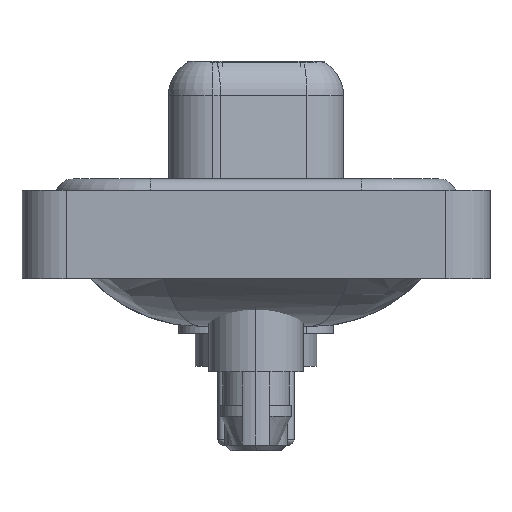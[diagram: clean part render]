
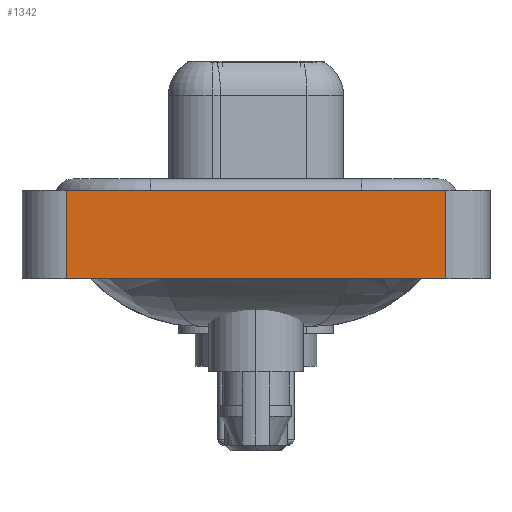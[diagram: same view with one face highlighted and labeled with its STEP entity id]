
A CAD part, left-side view. The second image highlights one B-rep face of the part: STEP entity #1342.
In plain terms, the highlighted planar face has unit normal (-1, 0, 0).
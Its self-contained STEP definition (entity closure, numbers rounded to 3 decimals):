
#61 = VERTEX_POINT ( 'NONE', #8482 ) ;
#891 = EDGE_LOOP ( 'NONE', ( #1955, #5107, #23149, #19632 ) ) ;
#1128 = EDGE_CURVE ( 'NONE', #61, #12502, #7749, .T. ) ;
#1342 = ADVANCED_FACE ( 'NONE', ( #24289 ), #12551, .T. ) ;
#1526 = VECTOR ( 'NONE', #23665, 1000. ) ;
#1574 = CARTESIAN_POINT ( 'NONE',  ( -7.35, -8.55, 0.4 ) ) ;
#1955 = ORIENTED_EDGE ( 'NONE', *, *, #8724, .T. ) ;
#3201 = CARTESIAN_POINT ( 'NONE',  ( -7.35, -8.55, -3.6 ) ) ;
#4560 = CARTESIAN_POINT ( 'NONE',  ( -7.35, 8.55, 0.4 ) ) ;
#4996 = LINE ( 'NONE', #3201, #21422 ) ;
#5107 = ORIENTED_EDGE ( 'NONE', *, *, #14108, .F. ) ;
#5480 = DIRECTION ( 'NONE',  ( 0., 0., 1. ) ) ;
#7309 = CARTESIAN_POINT ( 'NONE',  ( -7.35, -8.55, -3.6 ) ) ;
#7749 = LINE ( 'NONE', #10145, #1526 ) ;
#8010 = CARTESIAN_POINT ( 'NONE',  ( -7.35, -8.55, 0.4 ) ) ;
#8261 = LINE ( 'NONE', #8010, #17366 ) ;
#8482 = CARTESIAN_POINT ( 'NONE',  ( -7.35, 8.55, -3.6 ) ) ;
#8724 = EDGE_CURVE ( 'NONE', #21779, #14314, #4996, .T. ) ;
#10037 = DIRECTION ( 'NONE',  ( 0., -1., 0. ) ) ;
#10145 = CARTESIAN_POINT ( 'NONE',  ( -7.35, 8.55, -3.6 ) ) ;
#12502 = VERTEX_POINT ( 'NONE', #4560 ) ;
#12551 = PLANE ( 'NONE',  #16206 ) ;
#13520 = LINE ( 'NONE', #19129, #15244 ) ;
#14108 = EDGE_CURVE ( 'NONE', #12502, #14314, #8261, .T. ) ;
#14314 = VERTEX_POINT ( 'NONE', #1574 ) ;
#15244 = VECTOR ( 'NONE', #23342, 1000. ) ;
#16087 = EDGE_CURVE ( 'NONE', #61, #21779, #13520, .T. ) ;
#16206 = AXIS2_PLACEMENT_3D ( 'NONE', #22251, #16640, #24420 ) ;
#16640 = DIRECTION ( 'NONE',  ( -1., 0., 0. ) ) ;
#17366 = VECTOR ( 'NONE', #10037, 1000. ) ;
#19129 = CARTESIAN_POINT ( 'NONE',  ( -7.35, -8.55, -3.6 ) ) ;
#19632 = ORIENTED_EDGE ( 'NONE', *, *, #16087, .T. ) ;
#21422 = VECTOR ( 'NONE', #5480, 1000. ) ;
#21779 = VERTEX_POINT ( 'NONE', #7309 ) ;
#22251 = CARTESIAN_POINT ( 'NONE',  ( -7.35, -8.55, -3.6 ) ) ;
#23149 = ORIENTED_EDGE ( 'NONE', *, *, #1128, .F. ) ;
#23342 = DIRECTION ( 'NONE',  ( 0., -1., 0. ) ) ;
#23665 = DIRECTION ( 'NONE',  ( 0., 0., 1. ) ) ;
#24289 = FACE_OUTER_BOUND ( 'NONE', #891, .T. ) ;
#24420 = DIRECTION ( 'NONE',  ( 0., 0., 1. ) ) ;
